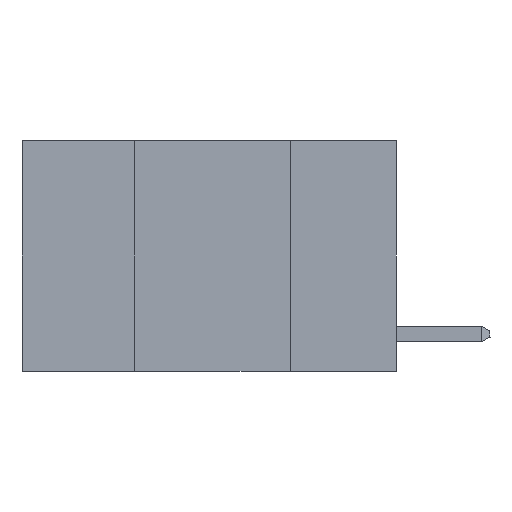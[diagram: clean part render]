
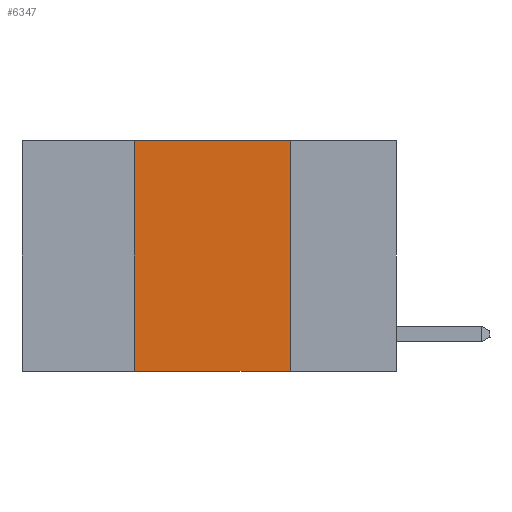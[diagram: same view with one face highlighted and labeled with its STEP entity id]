
A CAD part, left-side view. The second image highlights one B-rep face of the part: STEP entity #6347.
In plain terms, the highlighted planar face has unit normal (-1, 0, 0).
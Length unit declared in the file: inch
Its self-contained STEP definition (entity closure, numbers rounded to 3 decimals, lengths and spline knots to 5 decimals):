
#414 = FACE_OUTER_BOUND ( 'NONE', #2829, .T. ) ;
#481 = VERTEX_POINT ( 'NONE', #22960 ) ;
#730 = VECTOR ( 'NONE', #6448, 39.37008 ) ;
#1290 = DIRECTION ( 'NONE',  ( 0., 0., 1. ) ) ;
#2829 = EDGE_LOOP ( 'NONE', ( #14209, #11113, #8318, #12072 ) ) ;
#3040 = DIRECTION ( 'NONE',  ( 1., 0., 0. ) ) ;
#5295 = CARTESIAN_POINT ( 'NONE',  ( 0., 0.6, 0. ) ) ;
#5796 = EDGE_CURVE ( 'NONE', #15895, #481, #15130, .T. ) ;
#6261 = CARTESIAN_POINT ( 'NONE',  ( 0., 0.42, -0.37 ) ) ;
#6347 = ADVANCED_FACE ( 'NONE', ( #414 ), #13849, .F. ) ;
#6448 = DIRECTION ( 'NONE',  ( 0., 0., -1. ) ) ;
#6819 = LINE ( 'NONE', #5295, #12193 ) ;
#7376 = VECTOR ( 'NONE', #1290, 39.37008 ) ;
#7579 = AXIS2_PLACEMENT_3D ( 'NONE', #8436, #3040, #15669 ) ;
#7826 = EDGE_CURVE ( 'NONE', #18065, #481, #13922, .T. ) ;
#8318 = ORIENTED_EDGE ( 'NONE', *, *, #13457, .F. ) ;
#8436 = CARTESIAN_POINT ( 'NONE',  ( 0., 0.6, 0. ) ) ;
#10212 = CARTESIAN_POINT ( 'NONE',  ( 0., 0.6, -0.37 ) ) ;
#10297 = CARTESIAN_POINT ( 'NONE',  ( 0., 0.42, 0. ) ) ;
#11113 = ORIENTED_EDGE ( 'NONE', *, *, #18355, .F. ) ;
#12072 = ORIENTED_EDGE ( 'NONE', *, *, #7826, .T. ) ;
#12193 = VECTOR ( 'NONE', #17942, 39.37008 ) ;
#13023 = VERTEX_POINT ( 'NONE', #17968 ) ;
#13457 = EDGE_CURVE ( 'NONE', #18065, #13023, #21710, .T. ) ;
#13849 = PLANE ( 'NONE',  #7579 ) ;
#13922 = LINE ( 'NONE', #10212, #18727 ) ;
#14209 = ORIENTED_EDGE ( 'NONE', *, *, #5796, .F. ) ;
#15130 = LINE ( 'NONE', #19080, #730 ) ;
#15669 = DIRECTION ( 'NONE',  ( 0., 0., -1. ) ) ;
#15895 = VERTEX_POINT ( 'NONE', #23050 ) ;
#17942 = DIRECTION ( 'NONE',  ( 0., -1., 0. ) ) ;
#17968 = CARTESIAN_POINT ( 'NONE',  ( 0., 0.42, 0. ) ) ;
#18065 = VERTEX_POINT ( 'NONE', #6261 ) ;
#18355 = EDGE_CURVE ( 'NONE', #13023, #15895, #6819, .T. ) ;
#18727 = VECTOR ( 'NONE', #19190, 39.37008 ) ;
#19080 = CARTESIAN_POINT ( 'NONE',  ( 0., 0.17, 0. ) ) ;
#19190 = DIRECTION ( 'NONE',  ( 0., -1., 0. ) ) ;
#21710 = LINE ( 'NONE', #10297, #7376 ) ;
#22960 = CARTESIAN_POINT ( 'NONE',  ( 0., 0.17, -0.37 ) ) ;
#23050 = CARTESIAN_POINT ( 'NONE',  ( 0., 0.17, 0. ) ) ;
